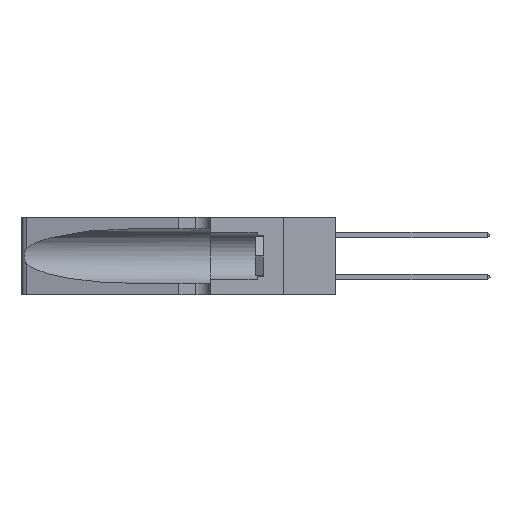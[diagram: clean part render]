
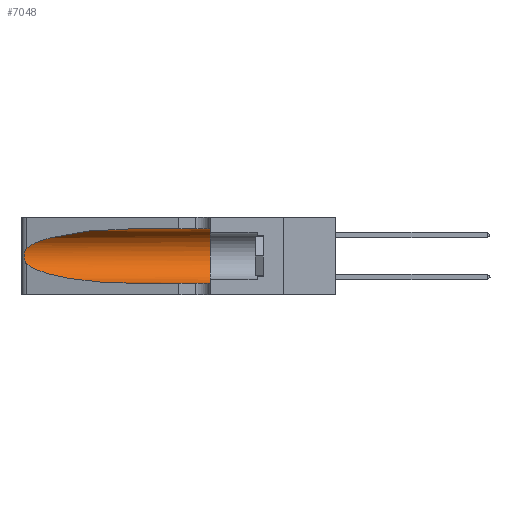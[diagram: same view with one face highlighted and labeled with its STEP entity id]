
A CAD part, left-side view. The second image highlights one B-rep face of the part: STEP entity #7048.
In plain terms, the highlighted cylindrical face has radius 3.308 mm (diameter 6.617 mm), a partial arc.
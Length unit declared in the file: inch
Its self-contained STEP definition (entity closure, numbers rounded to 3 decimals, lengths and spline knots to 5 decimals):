
#49 = CYLINDRICAL_SURFACE ( 'NONE', #39185, 0.13025 ) ;
#88 = CARTESIAN_POINT ( 'NONE',  ( 0.1305, 0.35, 0.185 ) ) ;
#171 = VECTOR ( 'NONE', #34566, 39.37008 ) ;
#1173 = ORIENTED_EDGE ( 'NONE', *, *, #4969, .F. ) ;
#2460 = DIRECTION ( 'NONE',  ( 0., -1., 0. ) ) ;
#4969 = EDGE_CURVE ( 'NONE', #39244, #10176, #9426, .T. ) ;
#4995 = CARTESIAN_POINT ( 'NONE',  ( 0.26018, 1.23835, 0.19895 ) ) ;
#6407 = DIRECTION ( 'NONE',  ( 0., 0., 1. ) ) ;
#6449 = VERTEX_POINT ( 'NONE', #17752 ) ;
#6610 = CARTESIAN_POINT ( 'NONE',  ( 0.25487, 1.22718, 0.22369 ) ) ;
#6934 = VERTEX_POINT ( 'NONE', #34295 ) ;
#7048 = ADVANCED_FACE ( 'NONE', ( #8801 ), #49, .F. ) ;
#8204 =( BOUNDED_CURVE ( )  B_SPLINE_CURVE ( 3, ( #37728, #14352, #11646, #11344 ),
 .UNSPECIFIED., .F., .F. ) 
 B_SPLINE_CURVE_WITH_KNOTS ( ( 4, 4 ),
 ( 3.44316, 4.71239 ),
 .UNSPECIFIED. ) 
 CURVE ( )  GEOMETRIC_REPRESENTATION_ITEM ( )  RATIONAL_B_SPLINE_CURVE ( ( 1., 0.87, 0.87, 1. ) ) 
 REPRESENTATION_ITEM ( '' )  );
#8801 = FACE_OUTER_BOUND ( 'NONE', #35902, .T. ) ;
#9111 = ORIENTED_EDGE ( 'NONE', *, *, #28917, .F. ) ;
#9426 = LINE ( 'NONE', #27576, #171 ) ;
#10051 = CARTESIAN_POINT ( 'NONE',  ( 0.1305, 0.72297, 0.31525 ) ) ;
#10176 = VERTEX_POINT ( 'NONE', #37788 ) ;
#10342 = AXIS2_PLACEMENT_3D ( 'NONE', #88, #39078, #6407 ) ;
#11344 = CARTESIAN_POINT ( 'NONE',  ( 0.1305, 0.72297, 0.05475 ) ) ;
#11539 = CIRCLE ( 'NONE', #10342, 0.13025 ) ;
#11646 = CARTESIAN_POINT ( 'NONE',  ( 0.18966, 0.96281, 0.05475 ) ) ;
#12382 = CARTESIAN_POINT ( 'NONE',  ( 0.2373, 1.15595, 0.28018 ) ) ;
#13190 = CARTESIAN_POINT ( 'NONE',  ( 0.25639, 1.23184, 0.21858 ) ) ;
#14352 = CARTESIAN_POINT ( 'NONE',  ( 0.2373, 1.15595, 0.08982 ) ) ;
#14681 = EDGE_CURVE ( 'NONE', #20133, #6449, #35398, .T. ) ;
#15568 = ORIENTED_EDGE ( 'NONE', *, *, #36455, .T. ) ;
#15658 = ORIENTED_EDGE ( 'NONE', *, *, #42098, .T. ) ;
#17752 = CARTESIAN_POINT ( 'NONE',  ( 0.25487, 1.22718, 0.14631 ) ) ;
#18518 = ORIENTED_EDGE ( 'NONE', *, *, #14681, .T. ) ;
#19167 = CARTESIAN_POINT ( 'NONE',  ( 0.25487, 1.22718, 0.22369 ) ) ;
#19404 = CARTESIAN_POINT ( 'NONE',  ( 0.26017, 1.23833, 0.17102 ) ) ;
#20133 = VERTEX_POINT ( 'NONE', #6610 ) ;
#20902 = CARTESIAN_POINT ( 'NONE',  ( 0.25789, 1.23486, 0.15765 ) ) ;
#21585 = ORIENTED_EDGE ( 'NONE', *, *, #27747, .T. ) ;
#22160 = CARTESIAN_POINT ( 'NONE',  ( 0.1305, 1.61858, 0.05475 ) ) ;
#26304 = CARTESIAN_POINT ( 'NONE',  ( 0.25555, 1.22993, 0.14849 ) ) ;
#27576 = CARTESIAN_POINT ( 'NONE',  ( 0.1305, 1.61858, 0.31525 ) ) ;
#27701 = CARTESIAN_POINT ( 'NONE',  ( 0.25787, 1.23484, 0.2124 ) ) ;
#27747 = EDGE_CURVE ( 'NONE', #6934, #33145, #39797, .T. ) ;
#27980 = CARTESIAN_POINT ( 'NONE',  ( 0.25487, 1.22718, 0.14631 ) ) ;
#28461 = CARTESIAN_POINT ( 'NONE',  ( 0.18966, 0.96281, 0.31525 ) ) ;
#28917 = EDGE_CURVE ( 'NONE', #10176, #33145, #11539, .T. ) ;
#29102 = VECTOR ( 'NONE', #2460, 39.37008 ) ;
#31585 = CARTESIAN_POINT ( 'NONE',  ( 0.1305, 0.72297, 0.31525 ) ) ;
#33058 = CARTESIAN_POINT ( 'NONE',  ( 0.25555, 1.22994, 0.2215 ) ) ;
#33145 = VERTEX_POINT ( 'NONE', #41718 ) ;
#33800 = CARTESIAN_POINT ( 'NONE',  ( 0.26075, 1.23896, 0.19203 ) ) ;
#34097 = CARTESIAN_POINT ( 'NONE',  ( 0.25854, 1.2359, 0.20912 ) ) ;
#34295 = CARTESIAN_POINT ( 'NONE',  ( 0.1305, 0.72297, 0.05475 ) ) ;
#34566 = DIRECTION ( 'NONE',  ( 0., -1., 0. ) ) ;
#34883 = CARTESIAN_POINT ( 'NONE',  ( 0.25487, 1.22718, 0.22369 ) ) ;
#35398 = B_SPLINE_CURVE_WITH_KNOTS ( 'NONE', 3,
 ( #19167, #33058, #13190, #27701, #34097, #4995, #33800, #35523, #19404, #39613, #20902, #41393, #26304, #27980 ),
 .UNSPECIFIED., .F., .F.,
 ( 4, 2, 2, 2, 2, 2, 4 ),
 ( 0., 0.00027, 0.00053, 0.00107, 0.0016, 0.00187, 0.00214 ),
 .UNSPECIFIED. ) ;
#35523 = CARTESIAN_POINT ( 'NONE',  ( 0.26075, 1.23896, 0.178 ) ) ;
#35792 = CARTESIAN_POINT ( 'NONE',  ( 0.1305, 1.61858, 0.185 ) ) ;
#35902 = EDGE_LOOP ( 'NONE', ( #15658, #18518, #15568, #21585, #9111, #1173 ) ) ;
#36455 = EDGE_CURVE ( 'NONE', #6449, #6934, #8204, .T. ) ;
#37728 = CARTESIAN_POINT ( 'NONE',  ( 0.25487, 1.22718, 0.14631 ) ) ;
#37788 = CARTESIAN_POINT ( 'NONE',  ( 0.1305, 0.35, 0.31525 ) ) ;
#38653 = DIRECTION ( 'NONE',  ( 0., 0., -1. ) ) ;
#38941 = DIRECTION ( 'NONE',  ( 0., -1., 0. ) ) ;
#39078 = DIRECTION ( 'NONE',  ( 0., 1., 0. ) ) ;
#39185 = AXIS2_PLACEMENT_3D ( 'NONE', #35792, #38941, #38653 ) ;
#39244 = VERTEX_POINT ( 'NONE', #10051 ) ;
#39613 = CARTESIAN_POINT ( 'NONE',  ( 0.25856, 1.23593, 0.16098 ) ) ;
#39796 =( BOUNDED_CURVE ( )  B_SPLINE_CURVE ( 3, ( #31585, #28461, #12382, #34883 ),
 .UNSPECIFIED., .F., .F. ) 
 B_SPLINE_CURVE_WITH_KNOTS ( ( 4, 4 ),
 ( 1.5708, 2.84003 ),
 .UNSPECIFIED. ) 
 CURVE ( )  GEOMETRIC_REPRESENTATION_ITEM ( )  RATIONAL_B_SPLINE_CURVE ( ( 1., 0.87, 0.87, 1. ) ) 
 REPRESENTATION_ITEM ( '' )  );
#39797 = LINE ( 'NONE', #22160, #29102 ) ;
#41393 = CARTESIAN_POINT ( 'NONE',  ( 0.25639, 1.23186, 0.15144 ) ) ;
#41718 = CARTESIAN_POINT ( 'NONE',  ( 0.1305, 0.35, 0.05475 ) ) ;
#42098 = EDGE_CURVE ( 'NONE', #39244, #20133, #39796, .T. ) ;
